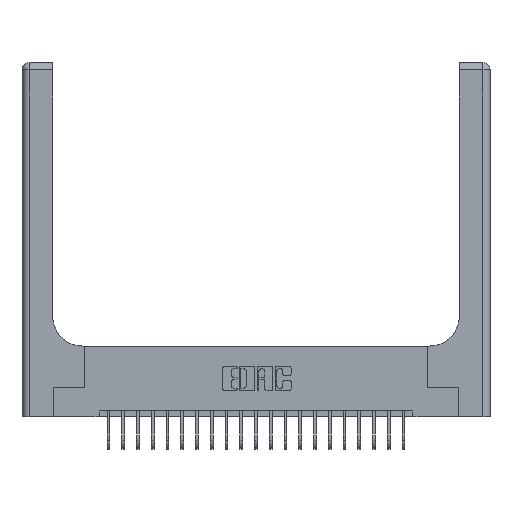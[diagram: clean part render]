
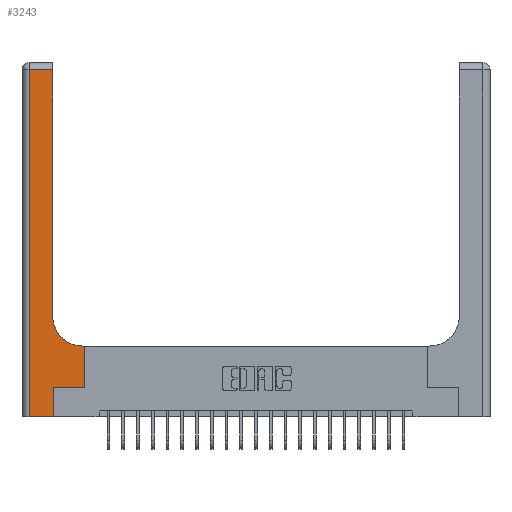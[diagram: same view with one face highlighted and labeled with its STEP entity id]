
A CAD part, top view. The second image highlights one B-rep face of the part: STEP entity #3243.
In plain terms, the highlighted planar face has unit normal (0, 0, 1).
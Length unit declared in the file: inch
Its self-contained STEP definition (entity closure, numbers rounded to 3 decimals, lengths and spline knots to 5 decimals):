
#11 = DIRECTION ( 'NONE',  ( 1., 0., 0. ) ) ;
#462 = PLANE ( 'NONE',  #10763 ) ;
#710 = ORIENTED_EDGE ( 'NONE', *, *, #6070, .T. ) ;
#770 = CARTESIAN_POINT ( 'NONE',  ( 0.06, 0., 0.37 ) ) ;
#1230 = DIRECTION ( 'NONE',  ( 0., 1., 0. ) ) ;
#1314 = EDGE_LOOP ( 'NONE', ( #710, #11414, #12206, #14276, #2710, #4161, #15337, #12002, #2946 ) ) ;
#1529 = VECTOR ( 'NONE', #19275, 39.37008 ) ;
#1950 = CARTESIAN_POINT ( 'NONE',  ( 0., 2.94, 0.37 ) ) ;
#2120 = CARTESIAN_POINT ( 'NONE',  ( 0.06, 2.94, 0.37 ) ) ;
#2364 = VECTOR ( 'NONE', #8436, 39.37008 ) ;
#2473 = CARTESIAN_POINT ( 'NONE',  ( 0.26, 0.85, 0.37 ) ) ;
#2710 = ORIENTED_EDGE ( 'NONE', *, *, #12881, .T. ) ;
#2859 = LINE ( 'NONE', #1950, #2364 ) ;
#2946 = ORIENTED_EDGE ( 'NONE', *, *, #3636, .T. ) ;
#3022 = CARTESIAN_POINT ( 'NONE',  ( 0.26, 3., 0.37 ) ) ;
#3196 = CARTESIAN_POINT ( 'NONE',  ( 0.265, 0.25, 0.37 ) ) ;
#3243 = ADVANCED_FACE ( 'NONE', ( #18402 ), #462, .F. ) ;
#3622 = VERTEX_POINT ( 'NONE', #21123 ) ;
#3636 = EDGE_CURVE ( 'NONE', #19892, #13793, #19946, .T. ) ;
#4036 = VERTEX_POINT ( 'NONE', #2120 ) ;
#4161 = ORIENTED_EDGE ( 'NONE', *, *, #9104, .T. ) ;
#4228 = LINE ( 'NONE', #3022, #21110 ) ;
#4294 = DIRECTION ( 'NONE',  ( 1., 0., 0. ) ) ;
#4570 = DIRECTION ( 'NONE',  ( 0., 1., 0. ) ) ;
#4593 = VERTEX_POINT ( 'NONE', #770 ) ;
#4644 = CARTESIAN_POINT ( 'NONE',  ( 0.528, 0.25, 0.37 ) ) ;
#4717 = EDGE_CURVE ( 'NONE', #4593, #17416, #17318, .T. ) ;
#4865 = VERTEX_POINT ( 'NONE', #4644 ) ;
#5308 = VECTOR ( 'NONE', #4294, 39.37008 ) ;
#5334 = DIRECTION ( 'NONE',  ( -1., 0., 0. ) ) ;
#6070 = EDGE_CURVE ( 'NONE', #13793, #16138, #4228, .T. ) ;
#8436 = DIRECTION ( 'NONE',  ( -1., 0., 0. ) ) ;
#9104 = EDGE_CURVE ( 'NONE', #3622, #4865, #17852, .T. ) ;
#9176 = EDGE_CURVE ( 'NONE', #4036, #4593, #12459, .T. ) ;
#9288 = CARTESIAN_POINT ( 'NONE',  ( 0.528, 0.25, 0.37 ) ) ;
#9684 = DIRECTION ( 'NONE',  ( 0., 0., -1. ) ) ;
#9914 = DIRECTION ( 'NONE',  ( 0., -1., 0. ) ) ;
#10763 = AXIS2_PLACEMENT_3D ( 'NONE', #11358, #15095, #5334 ) ;
#10787 = EDGE_CURVE ( 'NONE', #4865, #17538, #17533, .T. ) ;
#11310 = CARTESIAN_POINT ( 'NONE',  ( 0.51, 0.6, 0.37 ) ) ;
#11358 = CARTESIAN_POINT ( 'NONE',  ( 0., 3., 0.37 ) ) ;
#11414 = ORIENTED_EDGE ( 'NONE', *, *, #13161, .T. ) ;
#11564 = DIRECTION ( 'NONE',  ( -1., 0., 0. ) ) ;
#11928 = VECTOR ( 'NONE', #9914, 39.37008 ) ;
#12002 = ORIENTED_EDGE ( 'NONE', *, *, #16903, .T. ) ;
#12206 = ORIENTED_EDGE ( 'NONE', *, *, #9176, .T. ) ;
#12404 = CARTESIAN_POINT ( 'NONE',  ( 0., 0., 0.37 ) ) ;
#12459 = LINE ( 'NONE', #19555, #11928 ) ;
#12830 = LINE ( 'NONE', #14341, #16652 ) ;
#12881 = EDGE_CURVE ( 'NONE', #17416, #3622, #12830, .T. ) ;
#13161 = EDGE_CURVE ( 'NONE', #16138, #4036, #2859, .T. ) ;
#13793 = VERTEX_POINT ( 'NONE', #2473 ) ;
#14276 = ORIENTED_EDGE ( 'NONE', *, *, #4717, .T. ) ;
#14341 = CARTESIAN_POINT ( 'NONE',  ( 0.265, 0., 0.37 ) ) ;
#15095 = DIRECTION ( 'NONE',  ( 0., 0., -1. ) ) ;
#15337 = ORIENTED_EDGE ( 'NONE', *, *, #10787, .T. ) ;
#16138 = VERTEX_POINT ( 'NONE', #20585 ) ;
#16492 = VECTOR ( 'NONE', #1230, 39.37008 ) ;
#16507 = CARTESIAN_POINT ( 'NONE',  ( 0.528, 0.6, 0.37 ) ) ;
#16652 = VECTOR ( 'NONE', #4570, 39.37008 ) ;
#16903 = EDGE_CURVE ( 'NONE', #17538, #19892, #20939, .T. ) ;
#16973 = AXIS2_PLACEMENT_3D ( 'NONE', #19543, #9684, #11 ) ;
#17318 = LINE ( 'NONE', #12404, #5308 ) ;
#17416 = VERTEX_POINT ( 'NONE', #19237 ) ;
#17533 = LINE ( 'NONE', #9288, #16492 ) ;
#17538 = VERTEX_POINT ( 'NONE', #16507 ) ;
#17852 = LINE ( 'NONE', #3196, #1529 ) ;
#18115 = CARTESIAN_POINT ( 'NONE',  ( 0.26, 0.6, 0.37 ) ) ;
#18402 = FACE_OUTER_BOUND ( 'NONE', #1314, .T. ) ;
#19237 = CARTESIAN_POINT ( 'NONE',  ( 0.265, 0., 0.37 ) ) ;
#19275 = DIRECTION ( 'NONE',  ( 1., 0., 0. ) ) ;
#19383 = DIRECTION ( 'NONE',  ( 0., 1., 0. ) ) ;
#19543 = CARTESIAN_POINT ( 'NONE',  ( 0.51, 0.85, 0.37 ) ) ;
#19555 = CARTESIAN_POINT ( 'NONE',  ( 0.06, 3., 0.37 ) ) ;
#19892 = VERTEX_POINT ( 'NONE', #11310 ) ;
#19946 = CIRCLE ( 'NONE', #16973, 0.25 ) ;
#20432 = VECTOR ( 'NONE', #11564, 39.37008 ) ;
#20585 = CARTESIAN_POINT ( 'NONE',  ( 0.26, 2.94, 0.37 ) ) ;
#20939 = LINE ( 'NONE', #18115, #20432 ) ;
#21110 = VECTOR ( 'NONE', #19383, 39.37008 ) ;
#21123 = CARTESIAN_POINT ( 'NONE',  ( 0.265, 0.25, 0.37 ) ) ;
